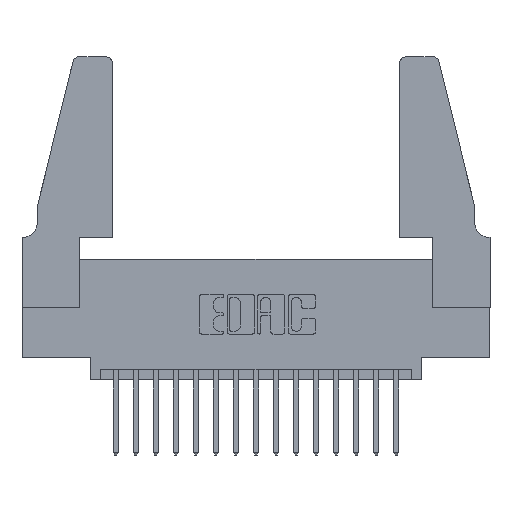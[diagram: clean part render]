
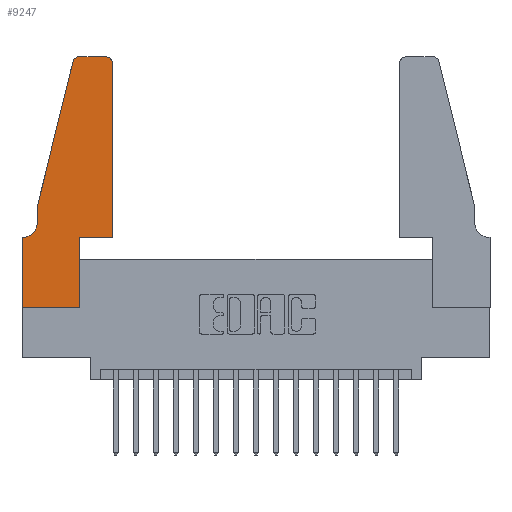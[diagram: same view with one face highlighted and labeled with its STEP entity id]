
A CAD part, top view. The second image highlights one B-rep face of the part: STEP entity #9247.
In plain terms, the highlighted planar face has unit normal (0, 0, 1).
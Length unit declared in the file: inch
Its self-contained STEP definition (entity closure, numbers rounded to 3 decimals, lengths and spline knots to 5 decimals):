
#104 = LINE ( 'NONE', #6102, #17029 ) ;
#459 = VERTEX_POINT ( 'NONE', #10873 ) ;
#477 = CARTESIAN_POINT ( 'NONE',  ( 0., 0., 0.37 ) ) ;
#647 = EDGE_LOOP ( 'NONE', ( #16703, #7687, #4151, #4942, #16769, #4989, #2325, #16201, #6438, #15258, #3499, #11241 ) ) ;
#743 = VERTEX_POINT ( 'NONE', #7062 ) ;
#857 = EDGE_CURVE ( 'NONE', #8098, #5625, #3777, .T. ) ;
#926 = CARTESIAN_POINT ( 'NONE',  ( 0., 0., 0.37 ) ) ;
#1407 = EDGE_CURVE ( 'NONE', #15243, #10110, #7021, .T. ) ;
#1742 = DIRECTION ( 'NONE',  ( 0., 1., 0. ) ) ;
#1854 = VECTOR ( 'NONE', #5129, 39.37008 ) ;
#2007 = CARTESIAN_POINT ( 'NONE',  ( 0.4205, 1.22, 0.37 ) ) ;
#2087 = CARTESIAN_POINT ( 'NONE',  ( 0., 0.35, 0.37 ) ) ;
#2224 = DIRECTION ( 'NONE',  ( -1., 0., 0. ) ) ;
#2325 = ORIENTED_EDGE ( 'NONE', *, *, #9027, .T. ) ;
#2452 = VERTEX_POINT ( 'NONE', #10977 ) ;
#2773 = VECTOR ( 'NONE', #10924, 39.37008 ) ;
#3108 = LINE ( 'NONE', #17133, #17067 ) ;
#3286 = LINE ( 'NONE', #6990, #13316 ) ;
#3457 = DIRECTION ( 'NONE',  ( 1., 0., 0. ) ) ;
#3499 = ORIENTED_EDGE ( 'NONE', *, *, #1407, .T. ) ;
#3777 = CIRCLE ( 'NONE', #9604, 0.07 ) ;
#4151 = ORIENTED_EDGE ( 'NONE', *, *, #4949, .T. ) ;
#4338 = CARTESIAN_POINT ( 'NONE',  ( 0.4505, 1.22, 0.37 ) ) ;
#4449 = VECTOR ( 'NONE', #9476, 39.37008 ) ;
#4508 = AXIS2_PLACEMENT_3D ( 'NONE', #6605, #7974, #17322 ) ;
#4599 = DIRECTION ( 'NONE',  ( 0., 0., 1. ) ) ;
#4942 = ORIENTED_EDGE ( 'NONE', *, *, #9325, .T. ) ;
#4949 = EDGE_CURVE ( 'NONE', #2452, #9091, #10123, .T. ) ;
#4989 = ORIENTED_EDGE ( 'NONE', *, *, #5977, .T. ) ;
#4993 = VERTEX_POINT ( 'NONE', #6889 ) ;
#5129 = DIRECTION ( 'NONE',  ( -1., 0., 0. ) ) ;
#5198 = EDGE_CURVE ( 'NONE', #14083, #2452, #7159, .T. ) ;
#5625 = VERTEX_POINT ( 'NONE', #8186 ) ;
#5756 = DIRECTION ( 'NONE',  ( 0., 1., 0. ) ) ;
#5977 = EDGE_CURVE ( 'NONE', #5625, #13065, #8837, .T. ) ;
#6102 = CARTESIAN_POINT ( 'NONE',  ( 0.4505, 0.35, 0.37 ) ) ;
#6185 = CARTESIAN_POINT ( 'NONE',  ( 0.4505, 0.35, 0.37 ) ) ;
#6438 = ORIENTED_EDGE ( 'NONE', *, *, #14359, .T. ) ;
#6575 = DIRECTION ( 'NONE',  ( 1., 0., 0. ) ) ;
#6605 = CARTESIAN_POINT ( 'NONE',  ( 0., 0.35, 0.37 ) ) ;
#6889 = CARTESIAN_POINT ( 'NONE',  ( 0.2865, 0.35, 0.37 ) ) ;
#6990 = CARTESIAN_POINT ( 'NONE',  ( 0.2865, 0.35, 0.37 ) ) ;
#7021 = LINE ( 'NONE', #11424, #16870 ) ;
#7062 = CARTESIAN_POINT ( 'NONE',  ( 0.4205, 1.25, 0.37 ) ) ;
#7159 = CIRCLE ( 'NONE', #8846, 0.03 ) ;
#7622 = VECTOR ( 'NONE', #6575, 39.37008 ) ;
#7687 = ORIENTED_EDGE ( 'NONE', *, *, #5198, .T. ) ;
#7974 = DIRECTION ( 'NONE',  ( 0., 0., 1. ) ) ;
#8098 = VERTEX_POINT ( 'NONE', #9450 ) ;
#8103 = CARTESIAN_POINT ( 'NONE',  ( 0.0755, 0.5, 0.37 ) ) ;
#8186 = CARTESIAN_POINT ( 'NONE',  ( 0.0055, 0.35, 0.37 ) ) ;
#8243 = CARTESIAN_POINT ( 'NONE',  ( 0.0055, 0.42, 0.37 ) ) ;
#8301 = DIRECTION ( 'NONE',  ( 0., 0., -1. ) ) ;
#8837 = LINE ( 'NONE', #17220, #1854 ) ;
#8846 = AXIS2_PLACEMENT_3D ( 'NONE', #12738, #4599, #14081 ) ;
#8951 = FACE_OUTER_BOUND ( 'NONE', #647, .T. ) ;
#9027 = EDGE_CURVE ( 'NONE', #13065, #459, #14641, .T. ) ;
#9038 = DIRECTION ( 'NONE',  ( -1., 0., 0. ) ) ;
#9091 = VERTEX_POINT ( 'NONE', #16989 ) ;
#9247 = ADVANCED_FACE ( 'NONE', ( #8951 ), #14689, .T. ) ;
#9325 = EDGE_CURVE ( 'NONE', #9091, #8098, #10849, .T. ) ;
#9450 = CARTESIAN_POINT ( 'NONE',  ( 0.0755, 0.42, 0.37 ) ) ;
#9476 = DIRECTION ( 'NONE',  ( 0., -1., 0. ) ) ;
#9604 = AXIS2_PLACEMENT_3D ( 'NONE', #8243, #8301, #9038 ) ;
#9806 = EDGE_CURVE ( 'NONE', #743, #14083, #3108, .T. ) ;
#10110 = VERTEX_POINT ( 'NONE', #4338 ) ;
#10123 = LINE ( 'NONE', #16230, #2773 ) ;
#10291 = AXIS2_PLACEMENT_3D ( 'NONE', #2007, #11655, #3457 ) ;
#10849 = LINE ( 'NONE', #8103, #4449 ) ;
#10873 = CARTESIAN_POINT ( 'NONE',  ( 0., 0., 0.37 ) ) ;
#10924 = DIRECTION ( 'NONE',  ( -0.239, -0.971, 0. ) ) ;
#10977 = CARTESIAN_POINT ( 'NONE',  ( 0.25487, 1.22718, 0.37 ) ) ;
#11079 = VECTOR ( 'NONE', #16825, 39.37008 ) ;
#11241 = ORIENTED_EDGE ( 'NONE', *, *, #14617, .T. ) ;
#11424 = CARTESIAN_POINT ( 'NONE',  ( 0.4505, 0.35, 0.37 ) ) ;
#11655 = DIRECTION ( 'NONE',  ( 0., 0., 1. ) ) ;
#12738 = CARTESIAN_POINT ( 'NONE',  ( 0.284, 1.22, 0.37 ) ) ;
#13065 = VERTEX_POINT ( 'NONE', #2087 ) ;
#13316 = VECTOR ( 'NONE', #5756, 39.37008 ) ;
#13327 = LINE ( 'NONE', #926, #7622 ) ;
#13895 = VERTEX_POINT ( 'NONE', #16677 ) ;
#14079 = EDGE_CURVE ( 'NONE', #459, #13895, #13327, .T. ) ;
#14081 = DIRECTION ( 'NONE',  ( 1., 0., 0. ) ) ;
#14083 = VERTEX_POINT ( 'NONE', #15991 ) ;
#14359 = EDGE_CURVE ( 'NONE', #13895, #4993, #3286, .T. ) ;
#14550 = EDGE_CURVE ( 'NONE', #4993, #15243, #104, .T. ) ;
#14617 = EDGE_CURVE ( 'NONE', #10110, #743, #16224, .T. ) ;
#14641 = LINE ( 'NONE', #477, #11079 ) ;
#14689 = PLANE ( 'NONE',  #4508 ) ;
#15243 = VERTEX_POINT ( 'NONE', #6185 ) ;
#15258 = ORIENTED_EDGE ( 'NONE', *, *, #14550, .T. ) ;
#15991 = CARTESIAN_POINT ( 'NONE',  ( 0.284, 1.25, 0.37 ) ) ;
#16201 = ORIENTED_EDGE ( 'NONE', *, *, #14079, .T. ) ;
#16224 = CIRCLE ( 'NONE', #10291, 0.03 ) ;
#16230 = CARTESIAN_POINT ( 'NONE',  ( 0.0755, 0.5, 0.37 ) ) ;
#16677 = CARTESIAN_POINT ( 'NONE',  ( 0.2865, 0., 0.37 ) ) ;
#16703 = ORIENTED_EDGE ( 'NONE', *, *, #9806, .T. ) ;
#16769 = ORIENTED_EDGE ( 'NONE', *, *, #857, .T. ) ;
#16825 = DIRECTION ( 'NONE',  ( 0., -1., 0. ) ) ;
#16834 = DIRECTION ( 'NONE',  ( 1., 0., 0. ) ) ;
#16870 = VECTOR ( 'NONE', #1742, 39.37008 ) ;
#16989 = CARTESIAN_POINT ( 'NONE',  ( 0.0755, 0.5, 0.37 ) ) ;
#17029 = VECTOR ( 'NONE', #16834, 39.37008 ) ;
#17067 = VECTOR ( 'NONE', #2224, 39.37008 ) ;
#17133 = CARTESIAN_POINT ( 'NONE',  ( 0.2605, 1.25, 0.37 ) ) ;
#17220 = CARTESIAN_POINT ( 'NONE',  ( 0.0755, 0.35, 0.37 ) ) ;
#17322 = DIRECTION ( 'NONE',  ( 1., 0., 0. ) ) ;
